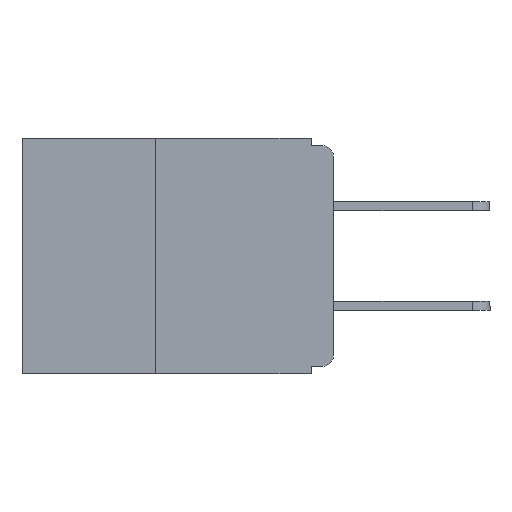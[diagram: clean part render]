
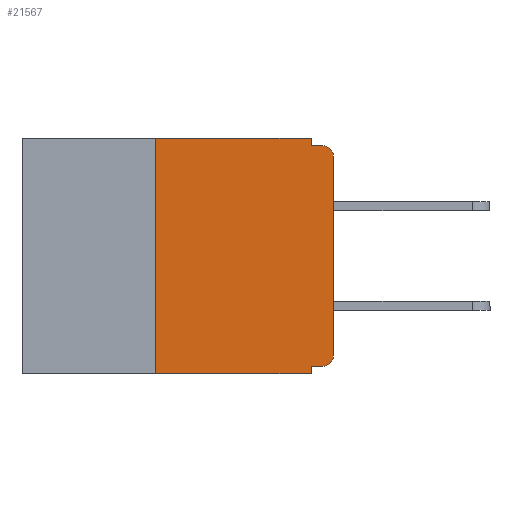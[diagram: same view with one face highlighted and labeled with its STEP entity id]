
A CAD part, left-side view. The second image highlights one B-rep face of the part: STEP entity #21567.
In plain terms, the highlighted planar face has unit normal (-1, 0, 0).
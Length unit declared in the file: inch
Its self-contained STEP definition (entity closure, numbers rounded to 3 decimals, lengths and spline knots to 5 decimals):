
#7 = EDGE_CURVE ( 'NONE', #15048, #5999, #21329, .T. ) ;
#239 = VECTOR ( 'NONE', #24603, 39.37008 ) ;
#559 = VERTEX_POINT ( 'NONE', #17504 ) ;
#695 = CARTESIAN_POINT ( 'NONE',  ( 0., 0.015, -0.32 ) ) ;
#822 = LINE ( 'NONE', #9989, #16634 ) ;
#1697 = ORIENTED_EDGE ( 'NONE', *, *, #11383, .F. ) ;
#2234 = VERTEX_POINT ( 'NONE', #10691 ) ;
#2865 = ORIENTED_EDGE ( 'NONE', *, *, #20674, .T. ) ;
#2881 = EDGE_CURVE ( 'NONE', #16991, #2234, #21241, .T. ) ;
#2910 = PLANE ( 'NONE',  #11203 ) ;
#3002 = VERTEX_POINT ( 'NONE', #24018 ) ;
#3843 = CARTESIAN_POINT ( 'NONE',  ( 0., 0., -0.01 ) ) ;
#4202 = DIRECTION ( 'NONE',  ( 0., -1., 0. ) ) ;
#4585 = ORIENTED_EDGE ( 'NONE', *, *, #8046, .F. ) ;
#5045 = DIRECTION ( 'NONE',  ( 1., 0., 0. ) ) ;
#5707 = EDGE_CURVE ( 'NONE', #15048, #18005, #23736, .T. ) ;
#5999 = VERTEX_POINT ( 'NONE', #24162 ) ;
#6094 = VECTOR ( 'NONE', #4202, 39.37008 ) ;
#6759 = LINE ( 'NONE', #22373, #6094 ) ;
#7197 = CARTESIAN_POINT ( 'NONE',  ( 0., 0.031, -0.33 ) ) ;
#7314 = DIRECTION ( 'NONE',  ( 0., -1., 0. ) ) ;
#7770 = ORIENTED_EDGE ( 'NONE', *, *, #7, .T. ) ;
#7781 = CARTESIAN_POINT ( 'NONE',  ( 0., 0.25, 0. ) ) ;
#7783 = VECTOR ( 'NONE', #21445, 39.37008 ) ;
#8046 = EDGE_CURVE ( 'NONE', #22102, #22962, #6759, .T. ) ;
#8098 = VECTOR ( 'NONE', #12252, 39.37008 ) ;
#9118 = ORIENTED_EDGE ( 'NONE', *, *, #12736, .T. ) ;
#9280 = CARTESIAN_POINT ( 'NONE',  ( 0., 0., -0.32 ) ) ;
#9464 = CARTESIAN_POINT ( 'NONE',  ( 0., 0.015, -0.025 ) ) ;
#9672 = ORIENTED_EDGE ( 'NONE', *, *, #2881, .T. ) ;
#9989 = CARTESIAN_POINT ( 'NONE',  ( 0., 0.25, -0.33 ) ) ;
#10691 = CARTESIAN_POINT ( 'NONE',  ( 0., 0.015, -0.01 ) ) ;
#10722 = CARTESIAN_POINT ( 'NONE',  ( 0., 0.031, 0. ) ) ;
#11203 = AXIS2_PLACEMENT_3D ( 'NONE', #17244, #5045, #19259 ) ;
#11299 = ORIENTED_EDGE ( 'NONE', *, *, #15443, .F. ) ;
#11306 = FACE_OUTER_BOUND ( 'NONE', #17553, .T. ) ;
#11378 = ORIENTED_EDGE ( 'NONE', *, *, #15293, .F. ) ;
#11383 = EDGE_CURVE ( 'NONE', #18005, #3002, #16793, .T. ) ;
#11410 = VECTOR ( 'NONE', #23244, 39.37008 ) ;
#12252 = DIRECTION ( 'NONE',  ( 0., -1., 0. ) ) ;
#12361 = DIRECTION ( 'NONE',  ( 0., 0., 1. ) ) ;
#12736 = EDGE_CURVE ( 'NONE', #559, #3002, #22601, .T. ) ;
#14089 = EDGE_CURVE ( 'NONE', #559, #22102, #822, .T. ) ;
#15048 = VERTEX_POINT ( 'NONE', #695 ) ;
#15293 = EDGE_CURVE ( 'NONE', #20807, #2234, #24031, .T. ) ;
#15443 = EDGE_CURVE ( 'NONE', #22962, #20807, #15452, .T. ) ;
#15452 = LINE ( 'NONE', #10722, #239 ) ;
#16001 = DIRECTION ( 'NONE',  ( -1., 0., 0. ) ) ;
#16060 = AXIS2_PLACEMENT_3D ( 'NONE', #18061, #16001, #16244 ) ;
#16097 = DIRECTION ( 'NONE',  ( 0., 0., 1. ) ) ;
#16244 = DIRECTION ( 'NONE',  ( 0., 0., -1. ) ) ;
#16634 = VECTOR ( 'NONE', #16097, 39.37008 ) ;
#16793 = LINE ( 'NONE', #7197, #11410 ) ;
#16991 = VERTEX_POINT ( 'NONE', #25982 ) ;
#17244 = CARTESIAN_POINT ( 'NONE',  ( 0., 0.437, 0. ) ) ;
#17394 = CARTESIAN_POINT ( 'NONE',  ( 0., 0.437, -0.33 ) ) ;
#17504 = CARTESIAN_POINT ( 'NONE',  ( 0., 0.25, -0.33 ) ) ;
#17553 = EDGE_LOOP ( 'NONE', ( #2865, #9672, #11378, #11299, #4585, #20972, #9118, #1697, #23221, #7770 ) ) ;
#18005 = VERTEX_POINT ( 'NONE', #25120 ) ;
#18061 = CARTESIAN_POINT ( 'NONE',  ( 0., 0.015, -0.305 ) ) ;
#18592 = LINE ( 'NONE', #26114, #23781 ) ;
#19259 = DIRECTION ( 'NONE',  ( 0., 0., -1. ) ) ;
#20674 = EDGE_CURVE ( 'NONE', #5999, #16991, #18592, .T. ) ;
#20807 = VERTEX_POINT ( 'NONE', #24628 ) ;
#20972 = ORIENTED_EDGE ( 'NONE', *, *, #14089, .F. ) ;
#21241 = CIRCLE ( 'NONE', #23855, 0.015 ) ;
#21329 = CIRCLE ( 'NONE', #16060, 0.015 ) ;
#21445 = DIRECTION ( 'NONE',  ( 0., 1., 0. ) ) ;
#21567 = ADVANCED_FACE ( 'NONE', ( #11306 ), #2910, .F. ) ;
#21999 = VECTOR ( 'NONE', #7314, 39.37008 ) ;
#22102 = VERTEX_POINT ( 'NONE', #7781 ) ;
#22373 = CARTESIAN_POINT ( 'NONE',  ( 0., 0.437, 0. ) ) ;
#22601 = LINE ( 'NONE', #17394, #21999 ) ;
#22962 = VERTEX_POINT ( 'NONE', #24403 ) ;
#23221 = ORIENTED_EDGE ( 'NONE', *, *, #5707, .F. ) ;
#23244 = DIRECTION ( 'NONE',  ( 0., 0., -1. ) ) ;
#23736 = LINE ( 'NONE', #9280, #7783 ) ;
#23781 = VECTOR ( 'NONE', #12361, 39.37008 ) ;
#23855 = AXIS2_PLACEMENT_3D ( 'NONE', #9464, #26188, #26126 ) ;
#24018 = CARTESIAN_POINT ( 'NONE',  ( 0., 0.031, -0.33 ) ) ;
#24031 = LINE ( 'NONE', #3843, #8098 ) ;
#24162 = CARTESIAN_POINT ( 'NONE',  ( 0., 0., -0.305 ) ) ;
#24403 = CARTESIAN_POINT ( 'NONE',  ( 0., 0.031, 0. ) ) ;
#24603 = DIRECTION ( 'NONE',  ( 0., 0., -1. ) ) ;
#24628 = CARTESIAN_POINT ( 'NONE',  ( 0., 0.031, -0.01 ) ) ;
#25120 = CARTESIAN_POINT ( 'NONE',  ( 0., 0.031, -0.32 ) ) ;
#25982 = CARTESIAN_POINT ( 'NONE',  ( 0., 0., -0.025 ) ) ;
#26114 = CARTESIAN_POINT ( 'NONE',  ( 0., 0., 0. ) ) ;
#26126 = DIRECTION ( 'NONE',  ( 0., 0., -1. ) ) ;
#26188 = DIRECTION ( 'NONE',  ( -1., 0., 0. ) ) ;
